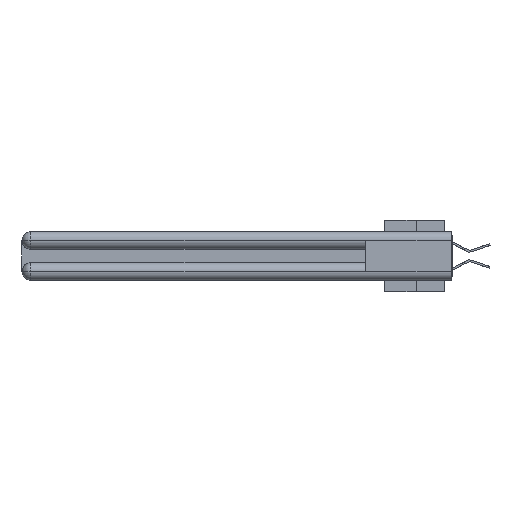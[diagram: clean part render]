
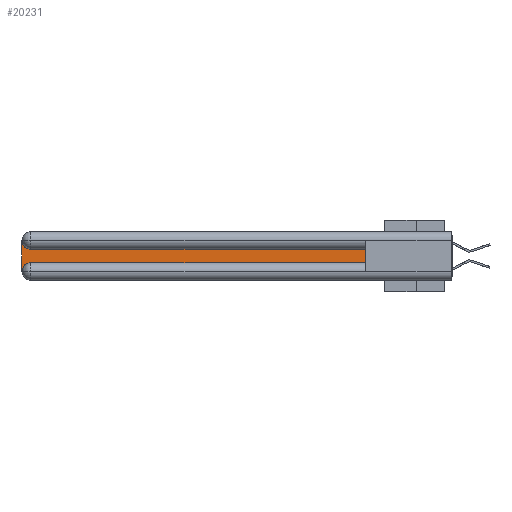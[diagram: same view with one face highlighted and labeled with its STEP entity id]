
A CAD part, left-side view. The second image highlights one B-rep face of the part: STEP entity #20231.
In plain terms, the highlighted planar face has unit normal (-1, 0, 0).
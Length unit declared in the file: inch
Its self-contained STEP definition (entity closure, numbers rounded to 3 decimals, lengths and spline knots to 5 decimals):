
#1517 = CIRCLE ( 'NONE', #21093, 0.06 ) ;
#2248 = LINE ( 'NONE', #19152, #29909 ) ;
#4883 = VECTOR ( 'NONE', #12014, 39.37008 ) ;
#6242 = CARTESIAN_POINT ( 'NONE',  ( 0.075, 3., -0.2175 ) ) ;
#6355 = CARTESIAN_POINT ( 'NONE',  ( 0.075, 3., -0.0625 ) ) ;
#6592 = EDGE_CURVE ( 'NONE', #27122, #31076, #1517, .T. ) ;
#7690 = ORIENTED_EDGE ( 'NONE', *, *, #34749, .T. ) ;
#8787 = EDGE_CURVE ( 'NONE', #31076, #17827, #31337, .T. ) ;
#10317 = DIRECTION ( 'NONE',  ( 1., 0., 0. ) ) ;
#12014 = DIRECTION ( 'NONE',  ( 0., 0., -1. ) ) ;
#13195 = CARTESIAN_POINT ( 'NONE',  ( 0.075, 0.6, -0.1225 ) ) ;
#13316 = VERTEX_POINT ( 'NONE', #25424 ) ;
#13817 = PLANE ( 'NONE',  #34779 ) ;
#15125 = ORIENTED_EDGE ( 'NONE', *, *, #35718, .T. ) ;
#15481 = VECTOR ( 'NONE', #24520, 39.37008 ) ;
#15775 = CARTESIAN_POINT ( 'NONE',  ( 0.075, 3., -0.2775 ) ) ;
#16585 = FACE_OUTER_BOUND ( 'NONE', #20120, .T. ) ;
#16772 = DIRECTION ( 'NONE',  ( 0., 0., -1. ) ) ;
#16827 = AXIS2_PLACEMENT_3D ( 'NONE', #35773, #10317, #29630 ) ;
#17640 = DIRECTION ( 'NONE',  ( 0., 0., -1. ) ) ;
#17827 = VERTEX_POINT ( 'NONE', #15775 ) ;
#18591 = CIRCLE ( 'NONE', #16827, 0.06 ) ;
#18924 = CARTESIAN_POINT ( 'NONE',  ( 0.075, 0.6, -0.2175 ) ) ;
#19152 = CARTESIAN_POINT ( 'NONE',  ( 0.075, 0.6, -0.2175 ) ) ;
#19694 = DIRECTION ( 'NONE',  ( 0., -1., 0. ) ) ;
#20120 = EDGE_LOOP ( 'NONE', ( #29015, #26825, #35573, #7690, #15125, #31585 ) ) ;
#20231 = ADVANCED_FACE ( 'NONE', ( #16585 ), #13817, .F. ) ;
#21093 = AXIS2_PLACEMENT_3D ( 'NONE', #25640, #34183, #17640 ) ;
#21945 = CARTESIAN_POINT ( 'NONE',  ( 0.075, 2.94, -0.2175 ) ) ;
#23119 = DIRECTION ( 'NONE',  ( 0., 0., 1. ) ) ;
#24520 = DIRECTION ( 'NONE',  ( 0., 1., 0. ) ) ;
#25424 = CARTESIAN_POINT ( 'NONE',  ( 0.075, 0.6, -0.1225 ) ) ;
#25640 = CARTESIAN_POINT ( 'NONE',  ( 0.075, 2.94, -0.0625 ) ) ;
#25695 = VERTEX_POINT ( 'NONE', #18924 ) ;
#26635 = CARTESIAN_POINT ( 'NONE',  ( 0.075, 0.6, -0.2175 ) ) ;
#26825 = ORIENTED_EDGE ( 'NONE', *, *, #6592, .T. ) ;
#27122 = VERTEX_POINT ( 'NONE', #34134 ) ;
#27314 = LINE ( 'NONE', #13195, #15481 ) ;
#27558 = DIRECTION ( 'NONE',  ( 1., 0., 0. ) ) ;
#29015 = ORIENTED_EDGE ( 'NONE', *, *, #32567, .T. ) ;
#29232 = EDGE_CURVE ( 'NONE', #25695, #13316, #31848, .T. ) ;
#29630 = DIRECTION ( 'NONE',  ( 0., 0., -1. ) ) ;
#29909 = VECTOR ( 'NONE', #19694, 39.37008 ) ;
#29936 = VERTEX_POINT ( 'NONE', #21945 ) ;
#30394 = VECTOR ( 'NONE', #23119, 39.37008 ) ;
#31076 = VERTEX_POINT ( 'NONE', #6355 ) ;
#31337 = LINE ( 'NONE', #6242, #4883 ) ;
#31585 = ORIENTED_EDGE ( 'NONE', *, *, #29232, .T. ) ;
#31848 = LINE ( 'NONE', #26635, #30394 ) ;
#32567 = EDGE_CURVE ( 'NONE', #13316, #27122, #27314, .T. ) ;
#34134 = CARTESIAN_POINT ( 'NONE',  ( 0.075, 2.94, -0.1225 ) ) ;
#34183 = DIRECTION ( 'NONE',  ( 1., 0., 0. ) ) ;
#34749 = EDGE_CURVE ( 'NONE', #17827, #29936, #18591, .T. ) ;
#34779 = AXIS2_PLACEMENT_3D ( 'NONE', #36103, #27558, #16772 ) ;
#35573 = ORIENTED_EDGE ( 'NONE', *, *, #8787, .T. ) ;
#35718 = EDGE_CURVE ( 'NONE', #29936, #25695, #2248, .T. ) ;
#35773 = CARTESIAN_POINT ( 'NONE',  ( 0.075, 2.94, -0.2775 ) ) ;
#36103 = CARTESIAN_POINT ( 'NONE',  ( 0.075, 3., -0.1225 ) ) ;
